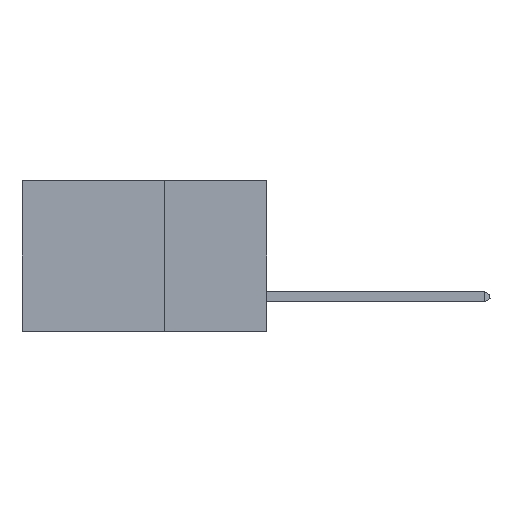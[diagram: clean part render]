
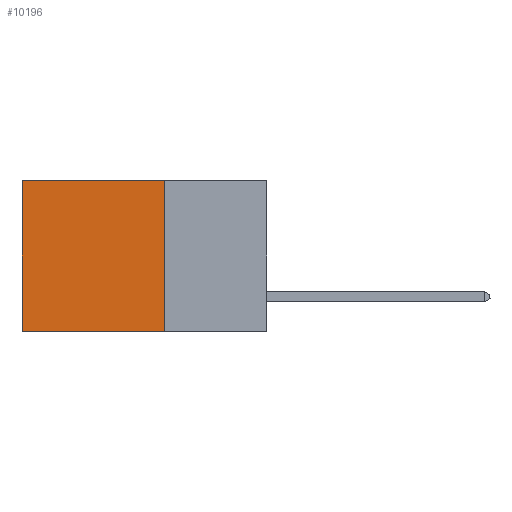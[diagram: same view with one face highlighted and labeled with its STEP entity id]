
A CAD part, left-side view. The second image highlights one B-rep face of the part: STEP entity #10196.
In plain terms, the highlighted planar face has unit normal (-1, 0, 0).
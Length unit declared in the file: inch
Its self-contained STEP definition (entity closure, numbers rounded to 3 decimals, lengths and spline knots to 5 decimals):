
#934 = PLANE ( 'NONE',  #11560 ) ;
#1079 = VECTOR ( 'NONE', #2967, 39.37008 ) ;
#1129 = CARTESIAN_POINT ( 'NONE',  ( 0.2875, 0.25, 0. ) ) ;
#1340 = CARTESIAN_POINT ( 'NONE',  ( 0.2875, 0.25, -0.37 ) ) ;
#1356 = LINE ( 'NONE', #14826, #11745 ) ;
#1748 = ORIENTED_EDGE ( 'NONE', *, *, #6866, .F. ) ;
#2345 = EDGE_LOOP ( 'NONE', ( #15798, #6086, #1748, #12887 ) ) ;
#2967 = DIRECTION ( 'NONE',  ( 0., 0., -1. ) ) ;
#3515 = CARTESIAN_POINT ( 'NONE',  ( 0.2875, 0.25, 0. ) ) ;
#3557 = VERTEX_POINT ( 'NONE', #6885 ) ;
#4802 = DIRECTION ( 'NONE',  ( 1., 0., 0. ) ) ;
#5168 = CARTESIAN_POINT ( 'NONE',  ( 0.2875, 0.6, -0.37 ) ) ;
#6086 = ORIENTED_EDGE ( 'NONE', *, *, #6610, .F. ) ;
#6610 = EDGE_CURVE ( 'NONE', #3557, #13134, #8903, .T. ) ;
#6866 = EDGE_CURVE ( 'NONE', #8554, #3557, #1356, .T. ) ;
#6885 = CARTESIAN_POINT ( 'NONE',  ( 0.2875, 0.25, -0.37 ) ) ;
#7079 = DIRECTION ( 'NONE',  ( 0., 0., -1. ) ) ;
#7887 = CARTESIAN_POINT ( 'NONE',  ( 0.2875, 0.25, 0. ) ) ;
#8410 = LINE ( 'NONE', #10783, #1079 ) ;
#8554 = VERTEX_POINT ( 'NONE', #7887 ) ;
#8903 = LINE ( 'NONE', #1340, #11965 ) ;
#8975 = DIRECTION ( 'NONE',  ( 0., 1., 0. ) ) ;
#10196 = ADVANCED_FACE ( 'NONE', ( #12271 ), #934, .F. ) ;
#10460 = DIRECTION ( 'NONE',  ( 0., 1., 0. ) ) ;
#10783 = CARTESIAN_POINT ( 'NONE',  ( 0.2875, 0.6, 0. ) ) ;
#11560 = AXIS2_PLACEMENT_3D ( 'NONE', #3515, #4802, #13903 ) ;
#11745 = VECTOR ( 'NONE', #7079, 39.37008 ) ;
#11965 = VECTOR ( 'NONE', #10460, 39.37008 ) ;
#12271 = FACE_OUTER_BOUND ( 'NONE', #2345, .T. ) ;
#12427 = EDGE_CURVE ( 'NONE', #8554, #12558, #15866, .T. ) ;
#12558 = VERTEX_POINT ( 'NONE', #13056 ) ;
#12887 = ORIENTED_EDGE ( 'NONE', *, *, #12427, .T. ) ;
#13056 = CARTESIAN_POINT ( 'NONE',  ( 0.2875, 0.6, 0. ) ) ;
#13134 = VERTEX_POINT ( 'NONE', #5168 ) ;
#13302 = EDGE_CURVE ( 'NONE', #12558, #13134, #8410, .T. ) ;
#13903 = DIRECTION ( 'NONE',  ( 0., 0., -1. ) ) ;
#14826 = CARTESIAN_POINT ( 'NONE',  ( 0.2875, 0.25, 0. ) ) ;
#15075 = VECTOR ( 'NONE', #8975, 39.37008 ) ;
#15798 = ORIENTED_EDGE ( 'NONE', *, *, #13302, .T. ) ;
#15866 = LINE ( 'NONE', #1129, #15075 ) ;
